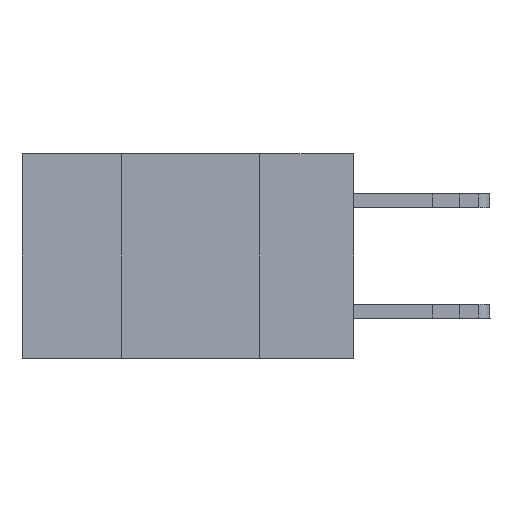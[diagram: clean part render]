
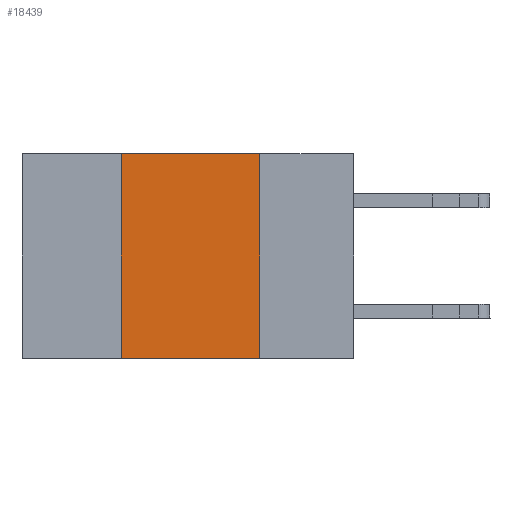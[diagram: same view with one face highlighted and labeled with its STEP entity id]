
A CAD part, left-side view. The second image highlights one B-rep face of the part: STEP entity #18439.
In plain terms, the highlighted planar face has unit normal (-1, 0, 0).
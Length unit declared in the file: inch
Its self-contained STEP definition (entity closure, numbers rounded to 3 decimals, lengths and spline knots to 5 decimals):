
#113 = EDGE_LOOP ( 'NONE', ( #7364, #3575, #9989, #8804 ) ) ;
#2627 = CARTESIAN_POINT ( 'NONE',  ( 0., 0.6, 0. ) ) ;
#2719 = VERTEX_POINT ( 'NONE', #3037 ) ;
#2735 = VERTEX_POINT ( 'NONE', #13304 ) ;
#3037 = CARTESIAN_POINT ( 'NONE',  ( 0., 0.17, -0.37 ) ) ;
#3493 = AXIS2_PLACEMENT_3D ( 'NONE', #14418, #16088, #6064 ) ;
#3575 = ORIENTED_EDGE ( 'NONE', *, *, #15003, .F. ) ;
#4125 = EDGE_CURVE ( 'NONE', #2735, #2719, #13396, .T. ) ;
#4186 = EDGE_CURVE ( 'NONE', #13497, #2719, #20136, .T. ) ;
#4260 = PLANE ( 'NONE',  #3493 ) ;
#4830 = CARTESIAN_POINT ( 'NONE',  ( 0., 0.6, -0.37 ) ) ;
#6064 = DIRECTION ( 'NONE',  ( 0., 0., -1. ) ) ;
#6525 = CARTESIAN_POINT ( 'NONE',  ( 0., 0.17, 0. ) ) ;
#6898 = DIRECTION ( 'NONE',  ( 0., 0., 1. ) ) ;
#7364 = ORIENTED_EDGE ( 'NONE', *, *, #4186, .F. ) ;
#8804 = ORIENTED_EDGE ( 'NONE', *, *, #4125, .T. ) ;
#8939 = VECTOR ( 'NONE', #21487, 39.37008 ) ;
#9989 = ORIENTED_EDGE ( 'NONE', *, *, #19420, .F. ) ;
#12907 = LINE ( 'NONE', #15245, #20664 ) ;
#13304 = CARTESIAN_POINT ( 'NONE',  ( 0., 0.42, -0.37 ) ) ;
#13396 = LINE ( 'NONE', #4830, #8939 ) ;
#13497 = VERTEX_POINT ( 'NONE', #6525 ) ;
#13536 = LINE ( 'NONE', #2627, #21301 ) ;
#13684 = FACE_OUTER_BOUND ( 'NONE', #113, .T. ) ;
#14418 = CARTESIAN_POINT ( 'NONE',  ( 0., 0.6, 0. ) ) ;
#15003 = EDGE_CURVE ( 'NONE', #15314, #13497, #13536, .T. ) ;
#15092 = CARTESIAN_POINT ( 'NONE',  ( 0., 0.17, 0. ) ) ;
#15161 = DIRECTION ( 'NONE',  ( 0., 0., -1. ) ) ;
#15245 = CARTESIAN_POINT ( 'NONE',  ( 0., 0.42, 0. ) ) ;
#15314 = VERTEX_POINT ( 'NONE', #16900 ) ;
#15774 = VECTOR ( 'NONE', #15161, 39.37008 ) ;
#16088 = DIRECTION ( 'NONE',  ( 1., 0., 0. ) ) ;
#16900 = CARTESIAN_POINT ( 'NONE',  ( 0., 0.42, 0. ) ) ;
#17876 = DIRECTION ( 'NONE',  ( 0., -1., 0. ) ) ;
#18439 = ADVANCED_FACE ( 'NONE', ( #13684 ), #4260, .F. ) ;
#19420 = EDGE_CURVE ( 'NONE', #2735, #15314, #12907, .T. ) ;
#20136 = LINE ( 'NONE', #15092, #15774 ) ;
#20664 = VECTOR ( 'NONE', #6898, 39.37008 ) ;
#21301 = VECTOR ( 'NONE', #17876, 39.37008 ) ;
#21487 = DIRECTION ( 'NONE',  ( 0., -1., 0. ) ) ;
